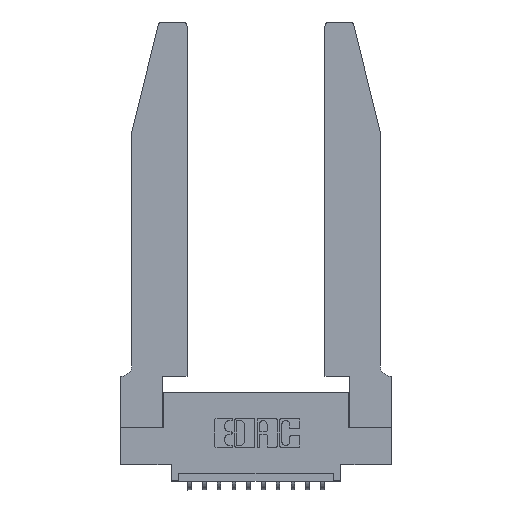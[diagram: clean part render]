
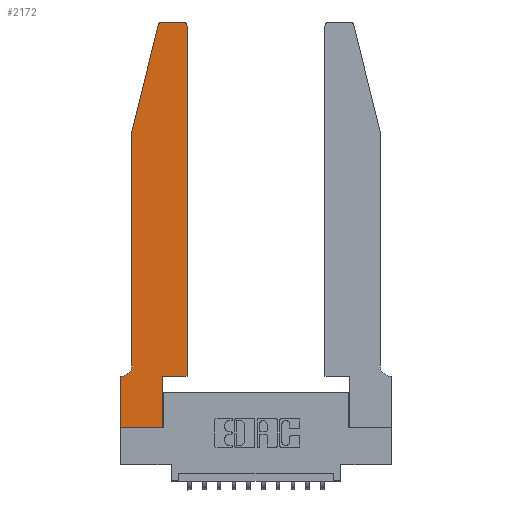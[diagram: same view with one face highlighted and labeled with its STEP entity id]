
A CAD part, top view. The second image highlights one B-rep face of the part: STEP entity #2172.
In plain terms, the highlighted planar face has unit normal (0, 0, 1).
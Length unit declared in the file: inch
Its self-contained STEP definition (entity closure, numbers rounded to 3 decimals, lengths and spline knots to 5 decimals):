
#486 = CARTESIAN_POINT ( 'NONE',  ( 0., 0.35, 0.37 ) ) ;
#1201 = VECTOR ( 'NONE', #15940, 39.37008 ) ;
#1264 = VECTOR ( 'NONE', #5861, 39.37008 ) ;
#1493 = DIRECTION ( 'NONE',  ( 0., 1., 0. ) ) ;
#1709 = CARTESIAN_POINT ( 'NONE',  ( 0.0055, 0.35, 0.37 ) ) ;
#1740 = CARTESIAN_POINT ( 'NONE',  ( 0.284, 2.72, 0.37 ) ) ;
#1893 = AXIS2_PLACEMENT_3D ( 'NONE', #13015, #16800, #8963 ) ;
#2013 = ORIENTED_EDGE ( 'NONE', *, *, #15486, .T. ) ;
#2172 = ADVANCED_FACE ( 'NONE', ( #11635 ), #5097, .T. ) ;
#2385 = DIRECTION ( 'NONE',  ( 0., -1., 0. ) ) ;
#2391 = AXIS2_PLACEMENT_3D ( 'NONE', #1740, #5547, #13177 ) ;
#2501 = CIRCLE ( 'NONE', #1893, 0.07 ) ;
#2675 = DIRECTION ( 'NONE',  ( 0., 0., 1. ) ) ;
#2733 = AXIS2_PLACEMENT_3D ( 'NONE', #3692, #16632, #16692 ) ;
#2972 = CARTESIAN_POINT ( 'NONE',  ( 0.4205, 2.75, 0.37 ) ) ;
#2979 = EDGE_CURVE ( 'NONE', #11945, #10904, #5077, .T. ) ;
#3292 = LINE ( 'NONE', #4569, #11643 ) ;
#3653 = CARTESIAN_POINT ( 'NONE',  ( 0.2605, 2.75, 0.37 ) ) ;
#3692 = CARTESIAN_POINT ( 'NONE',  ( 0., 0.35, 0.37 ) ) ;
#3731 = EDGE_CURVE ( 'NONE', #12176, #14604, #7333, .T. ) ;
#3758 = AXIS2_PLACEMENT_3D ( 'NONE', #13098, #2675, #13271 ) ;
#3825 = CARTESIAN_POINT ( 'NONE',  ( 0.0755, 0.42, 0.37 ) ) ;
#4049 = CARTESIAN_POINT ( 'NONE',  ( 0.0755, 2., 0.37 ) ) ;
#4053 = ORIENTED_EDGE ( 'NONE', *, *, #13083, .T. ) ;
#4256 = VERTEX_POINT ( 'NONE', #11895 ) ;
#4372 = CARTESIAN_POINT ( 'NONE',  ( 0.0755, 2., 0.37 ) ) ;
#4501 = EDGE_CURVE ( 'NONE', #12953, #13135, #12984, .T. ) ;
#4569 = CARTESIAN_POINT ( 'NONE',  ( 0.2865, 0.35, 0.37 ) ) ;
#4685 = EDGE_CURVE ( 'NONE', #13527, #4256, #5643, .T. ) ;
#5044 = DIRECTION ( 'NONE',  ( 1., 0., 0. ) ) ;
#5077 = LINE ( 'NONE', #11710, #16676 ) ;
#5097 = PLANE ( 'NONE',  #2733 ) ;
#5547 = DIRECTION ( 'NONE',  ( 0., 0., 1. ) ) ;
#5571 = ORIENTED_EDGE ( 'NONE', *, *, #9324, .T. ) ;
#5643 = LINE ( 'NONE', #3653, #10334 ) ;
#5649 = VECTOR ( 'NONE', #8445, 39.37008 ) ;
#5861 = DIRECTION ( 'NONE',  ( 1., 0., 0. ) ) ;
#6710 = ORIENTED_EDGE ( 'NONE', *, *, #16524, .T. ) ;
#7221 = EDGE_CURVE ( 'NONE', #16740, #12176, #9650, .T. ) ;
#7333 = LINE ( 'NONE', #16109, #14843 ) ;
#7394 = CARTESIAN_POINT ( 'NONE',  ( 0.2865, 0., 0.37 ) ) ;
#7426 = ORIENTED_EDGE ( 'NONE', *, *, #4685, .T. ) ;
#7449 = CARTESIAN_POINT ( 'NONE',  ( 0.4505, 2.72, 0.37 ) ) ;
#8006 = CARTESIAN_POINT ( 'NONE',  ( 0.25487, 2.72718, 0.37 ) ) ;
#8157 = LINE ( 'NONE', #8477, #1264 ) ;
#8212 = CARTESIAN_POINT ( 'NONE',  ( 0.4505, 0.35, 0.37 ) ) ;
#8445 = DIRECTION ( 'NONE',  ( -0.239, -0.971, 0. ) ) ;
#8477 = CARTESIAN_POINT ( 'NONE',  ( 0., 0., 0.37 ) ) ;
#8653 = DIRECTION ( 'NONE',  ( 0., 1., 0. ) ) ;
#8803 = DIRECTION ( 'NONE',  ( -1., 0., 0. ) ) ;
#8963 = DIRECTION ( 'NONE',  ( -1., 0., 0. ) ) ;
#9067 = CARTESIAN_POINT ( 'NONE',  ( 0., 0., 0.37 ) ) ;
#9098 = LINE ( 'NONE', #4372, #5649 ) ;
#9324 = EDGE_CURVE ( 'NONE', #16393, #16740, #3292, .T. ) ;
#9339 = EDGE_CURVE ( 'NONE', #14805, #16393, #8157, .T. ) ;
#9650 = LINE ( 'NONE', #14258, #14356 ) ;
#10016 = ORIENTED_EDGE ( 'NONE', *, *, #3731, .T. ) ;
#10145 = CIRCLE ( 'NONE', #2391, 0.03 ) ;
#10249 = ORIENTED_EDGE ( 'NONE', *, *, #7221, .T. ) ;
#10334 = VECTOR ( 'NONE', #8803, 39.37008 ) ;
#10375 = EDGE_LOOP ( 'NONE', ( #7426, #10938, #11312, #12574, #6710, #10814, #4053, #16295, #5571, #10249, #10016, #2013 ) ) ;
#10814 = ORIENTED_EDGE ( 'NONE', *, *, #2979, .T. ) ;
#10904 = VERTEX_POINT ( 'NONE', #486 ) ;
#10938 = ORIENTED_EDGE ( 'NONE', *, *, #12167, .T. ) ;
#11142 = LINE ( 'NONE', #16654, #14007 ) ;
#11312 = ORIENTED_EDGE ( 'NONE', *, *, #11452, .T. ) ;
#11452 = EDGE_CURVE ( 'NONE', #14287, #12953, #9098, .T. ) ;
#11635 = FACE_OUTER_BOUND ( 'NONE', #10375, .T. ) ;
#11643 = VECTOR ( 'NONE', #8653, 39.37008 ) ;
#11710 = CARTESIAN_POINT ( 'NONE',  ( 0.0755, 0.35, 0.37 ) ) ;
#11895 = CARTESIAN_POINT ( 'NONE',  ( 0.284, 2.75, 0.37 ) ) ;
#11945 = VERTEX_POINT ( 'NONE', #1709 ) ;
#12167 = EDGE_CURVE ( 'NONE', #4256, #14287, #10145, .T. ) ;
#12176 = VERTEX_POINT ( 'NONE', #8212 ) ;
#12507 = CIRCLE ( 'NONE', #3758, 0.03 ) ;
#12574 = ORIENTED_EDGE ( 'NONE', *, *, #4501, .T. ) ;
#12953 = VERTEX_POINT ( 'NONE', #4049 ) ;
#12984 = LINE ( 'NONE', #16104, #1201 ) ;
#13015 = CARTESIAN_POINT ( 'NONE',  ( 0.0055, 0.42, 0.37 ) ) ;
#13083 = EDGE_CURVE ( 'NONE', #10904, #14805, #11142, .T. ) ;
#13098 = CARTESIAN_POINT ( 'NONE',  ( 0.4205, 2.72, 0.37 ) ) ;
#13135 = VERTEX_POINT ( 'NONE', #3825 ) ;
#13177 = DIRECTION ( 'NONE',  ( 1., 0., 0. ) ) ;
#13271 = DIRECTION ( 'NONE',  ( 1., 0., 0. ) ) ;
#13527 = VERTEX_POINT ( 'NONE', #2972 ) ;
#13593 = CARTESIAN_POINT ( 'NONE',  ( 0.2865, 0.35, 0.37 ) ) ;
#14007 = VECTOR ( 'NONE', #2385, 39.37008 ) ;
#14258 = CARTESIAN_POINT ( 'NONE',  ( 0.4505, 0.35, 0.37 ) ) ;
#14287 = VERTEX_POINT ( 'NONE', #8006 ) ;
#14356 = VECTOR ( 'NONE', #5044, 39.37008 ) ;
#14604 = VERTEX_POINT ( 'NONE', #7449 ) ;
#14805 = VERTEX_POINT ( 'NONE', #9067 ) ;
#14843 = VECTOR ( 'NONE', #1493, 39.37008 ) ;
#15486 = EDGE_CURVE ( 'NONE', #14604, #13527, #12507, .T. ) ;
#15940 = DIRECTION ( 'NONE',  ( 0., -1., 0. ) ) ;
#16053 = DIRECTION ( 'NONE',  ( -1., 0., 0. ) ) ;
#16104 = CARTESIAN_POINT ( 'NONE',  ( 0.0755, 2., 0.37 ) ) ;
#16109 = CARTESIAN_POINT ( 'NONE',  ( 0.4505, 0.35, 0.37 ) ) ;
#16295 = ORIENTED_EDGE ( 'NONE', *, *, #9339, .T. ) ;
#16393 = VERTEX_POINT ( 'NONE', #7394 ) ;
#16524 = EDGE_CURVE ( 'NONE', #13135, #11945, #2501, .T. ) ;
#16632 = DIRECTION ( 'NONE',  ( 0., 0., 1. ) ) ;
#16654 = CARTESIAN_POINT ( 'NONE',  ( 0., 0., 0.37 ) ) ;
#16676 = VECTOR ( 'NONE', #16053, 39.37008 ) ;
#16692 = DIRECTION ( 'NONE',  ( 1., 0., 0. ) ) ;
#16740 = VERTEX_POINT ( 'NONE', #13593 ) ;
#16800 = DIRECTION ( 'NONE',  ( 0., 0., -1. ) ) ;
